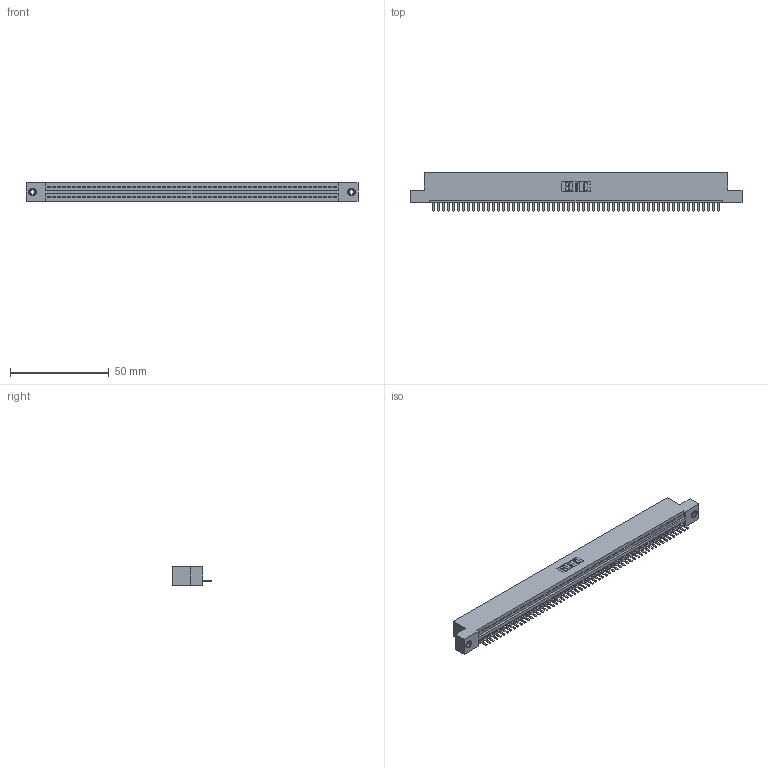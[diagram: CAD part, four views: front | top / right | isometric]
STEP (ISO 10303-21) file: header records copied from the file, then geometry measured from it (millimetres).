
FILE_DESCRIPTION (( 'STEP AP203' ), '1' );
FILE_NAME ('395-058-520-108.STEP', '2018-11-22T23:57:43', ( '' ), ( '' ), 'SwSTEP 2.0', 'SolidWorks 2016', '' );
FILE_SCHEMA (( 'CONFIG_CONTROL_DESIGN' ));
Length unit declared in the file: inch
Products named in the file (4): 345-250-001_345-250-003-102; 345-292-001_345-293-120; 345 Part_Flush Mounting Lugs - 0.156 Dia-TI; 395-058-520-108
Assembly tree (61 placements, depth 2):
  395-058-520-108
    345 Part_Flush Mounting Lugs - 0.156 Dia-TI
    345-292-001_345-293-120  x58
    345-250-001_345-250-003-102  x2
Bounding box: 168.53 x 19.68 x 9.4 mm (x, y, z)
Volume: 15964.8 mm3; surface area: 20906.5 mm2
Topology: 61 solids, 61 shells, 3782 faces, 11149 edges, 7270 vertices
Faces by surface type: plane 2548, cylinder 1218, cone 12, torus 4
Entity records: 42798 total; most frequent: CARTESIAN_POINT 7405, ORIENTED_EDGE 7378, DIRECTION 6459, EDGE_CURVE 3689, VECTOR 3301, LINE 3301, VERTEX_POINT 2452, AXIS2_PLACEMENT_3D 1579
